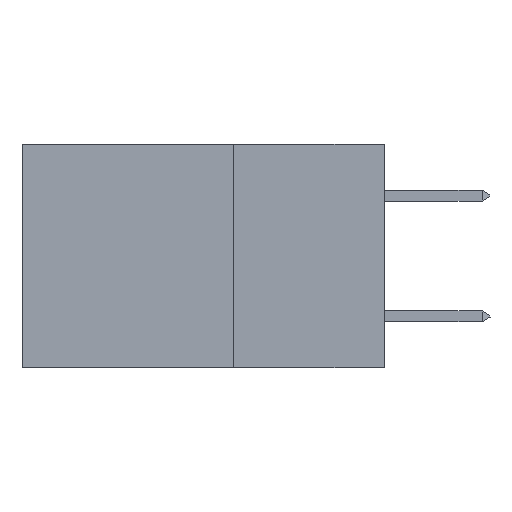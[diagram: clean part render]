
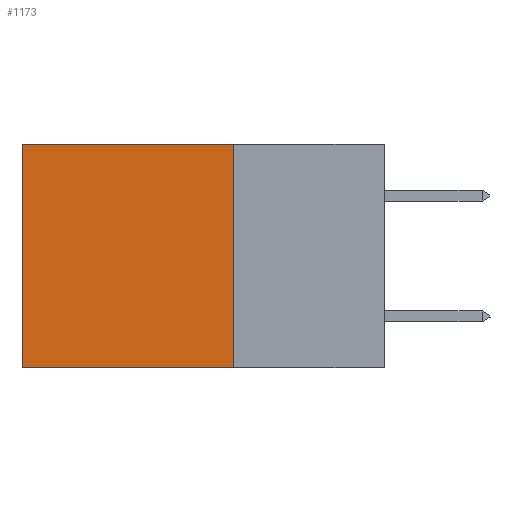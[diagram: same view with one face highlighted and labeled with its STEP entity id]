
A CAD part, left-side view. The second image highlights one B-rep face of the part: STEP entity #1173.
In plain terms, the highlighted planar face has unit normal (-1, 0, 0).
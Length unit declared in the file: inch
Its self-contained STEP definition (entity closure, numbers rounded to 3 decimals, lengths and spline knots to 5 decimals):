
#8 = ORIENTED_EDGE ( 'NONE', *, *, #5743, .F. ) ;
#76 = VERTEX_POINT ( 'NONE', #12963 ) ;
#384 = CARTESIAN_POINT ( 'NONE',  ( 0.2875, 0.25, 0. ) ) ;
#387 = DIRECTION ( 'NONE',  ( 0., 0., -1. ) ) ;
#1173 = ADVANCED_FACE ( 'NONE', ( #4522 ), #18792, .F. ) ;
#2224 = DIRECTION ( 'NONE',  ( 0., 0., -1. ) ) ;
#2328 = CARTESIAN_POINT ( 'NONE',  ( 0.2875, 0.25, 0. ) ) ;
#2728 = EDGE_CURVE ( 'NONE', #76, #23275, #8072, .T. ) ;
#3390 = VECTOR ( 'NONE', #16200, 39.37008 ) ;
#3396 = DIRECTION ( 'NONE',  ( 0., 1., 0. ) ) ;
#3436 = VERTEX_POINT ( 'NONE', #19967 ) ;
#3922 = CARTESIAN_POINT ( 'NONE',  ( 0.2875, 0.6, -0.37 ) ) ;
#4096 = VECTOR ( 'NONE', #2224, 39.37008 ) ;
#4522 = FACE_OUTER_BOUND ( 'NONE', #17855, .T. ) ;
#5743 = EDGE_CURVE ( 'NONE', #9182, #76, #16655, .T. ) ;
#6049 = CARTESIAN_POINT ( 'NONE',  ( 0.2875, 0.25, -0.37 ) ) ;
#8072 = LINE ( 'NONE', #6049, #17296 ) ;
#8886 = CARTESIAN_POINT ( 'NONE',  ( 0.2875, 0.6, 0. ) ) ;
#9182 = VERTEX_POINT ( 'NONE', #384 ) ;
#12963 = CARTESIAN_POINT ( 'NONE',  ( 0.2875, 0.25, -0.37 ) ) ;
#13279 = CARTESIAN_POINT ( 'NONE',  ( 0.2875, 0.25, 0. ) ) ;
#13346 = DIRECTION ( 'NONE',  ( 0., 1., 0. ) ) ;
#13634 = DIRECTION ( 'NONE',  ( 1., 0., 0. ) ) ;
#13862 = ORIENTED_EDGE ( 'NONE', *, *, #20835, .T. ) ;
#13990 = ORIENTED_EDGE ( 'NONE', *, *, #2728, .F. ) ;
#14549 = LINE ( 'NONE', #19837, #20911 ) ;
#14645 = EDGE_CURVE ( 'NONE', #3436, #23275, #17993, .T. ) ;
#16200 = DIRECTION ( 'NONE',  ( 0., 0., -1. ) ) ;
#16655 = LINE ( 'NONE', #13279, #4096 ) ;
#17296 = VECTOR ( 'NONE', #13346, 39.37008 ) ;
#17855 = EDGE_LOOP ( 'NONE', ( #22602, #13990, #8, #13862 ) ) ;
#17993 = LINE ( 'NONE', #8886, #3390 ) ;
#18047 = AXIS2_PLACEMENT_3D ( 'NONE', #2328, #13634, #387 ) ;
#18792 = PLANE ( 'NONE',  #18047 ) ;
#19837 = CARTESIAN_POINT ( 'NONE',  ( 0.2875, 0.25, 0. ) ) ;
#19967 = CARTESIAN_POINT ( 'NONE',  ( 0.2875, 0.6, 0. ) ) ;
#20835 = EDGE_CURVE ( 'NONE', #9182, #3436, #14549, .T. ) ;
#20911 = VECTOR ( 'NONE', #3396, 39.37008 ) ;
#22602 = ORIENTED_EDGE ( 'NONE', *, *, #14645, .T. ) ;
#23275 = VERTEX_POINT ( 'NONE', #3922 ) ;
